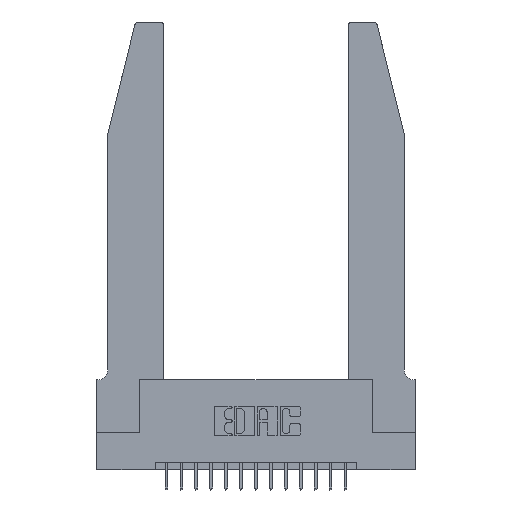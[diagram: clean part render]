
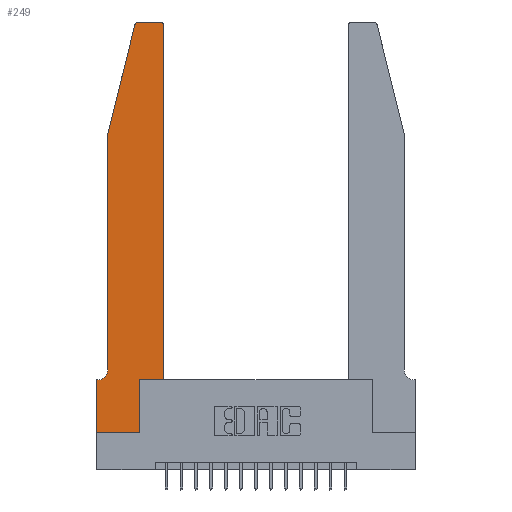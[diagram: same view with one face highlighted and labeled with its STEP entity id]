
A CAD part, top view. The second image highlights one B-rep face of the part: STEP entity #249.
In plain terms, the highlighted planar face has unit normal (0, 0, 1).
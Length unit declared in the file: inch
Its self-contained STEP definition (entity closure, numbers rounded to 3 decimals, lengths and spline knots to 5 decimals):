
#40 = CARTESIAN_POINT ( 'NONE',  ( 0., 0.35, 0.37 ) ) ;
#49 = ORIENTED_EDGE ( 'NONE', *, *, #11811, .T. ) ;
#57 = EDGE_CURVE ( 'NONE', #17818, #14148, #18195, .T. ) ;
#115 = EDGE_CURVE ( 'NONE', #15744, #13533, #5844, .T. ) ;
#156 = LINE ( 'NONE', #17797, #12013 ) ;
#249 = ADVANCED_FACE ( 'NONE', ( #4675 ), #346, .T. ) ;
#346 = PLANE ( 'NONE',  #12127 ) ;
#820 = VECTOR ( 'NONE', #7299, 39.37008 ) ;
#1170 = VERTEX_POINT ( 'NONE', #18199 ) ;
#1199 = ORIENTED_EDGE ( 'NONE', *, *, #8358, .T. ) ;
#1574 = CARTESIAN_POINT ( 'NONE',  ( 0.4205, 2.72, 0.37 ) ) ;
#1672 = VECTOR ( 'NONE', #6072, 39.37008 ) ;
#1860 = DIRECTION ( 'NONE',  ( 0., 0., 1. ) ) ;
#2452 = CARTESIAN_POINT ( 'NONE',  ( 0.4505, 0.35, 0.37 ) ) ;
#2607 = CIRCLE ( 'NONE', #3213, 0.07 ) ;
#2628 = CARTESIAN_POINT ( 'NONE',  ( 0.2865, 0.35, 0.37 ) ) ;
#2839 = ORIENTED_EDGE ( 'NONE', *, *, #11346, .T. ) ;
#3213 = AXIS2_PLACEMENT_3D ( 'NONE', #11190, #4967, #5063 ) ;
#3426 = DIRECTION ( 'NONE',  ( -1., 0., 0. ) ) ;
#3607 = VERTEX_POINT ( 'NONE', #10942 ) ;
#4304 = CARTESIAN_POINT ( 'NONE',  ( 0.0755, 0.35, 0.37 ) ) ;
#4504 = VECTOR ( 'NONE', #15338, 39.37008 ) ;
#4586 = DIRECTION ( 'NONE',  ( 0., -1., 0. ) ) ;
#4675 = FACE_OUTER_BOUND ( 'NONE', #10926, .T. ) ;
#4815 = CARTESIAN_POINT ( 'NONE',  ( 0.4505, 0.35, 0.37 ) ) ;
#4860 = VECTOR ( 'NONE', #8198, 39.37008 ) ;
#4967 = DIRECTION ( 'NONE',  ( 0., 0., -1. ) ) ;
#5063 = DIRECTION ( 'NONE',  ( -1., 0., 0. ) ) ;
#5079 = VECTOR ( 'NONE', #5709, 39.37008 ) ;
#5249 = LINE ( 'NONE', #2452, #4860 ) ;
#5508 = CARTESIAN_POINT ( 'NONE',  ( 0.284, 2.75, 0.37 ) ) ;
#5709 = DIRECTION ( 'NONE',  ( 0., 1., 0. ) ) ;
#5743 = CARTESIAN_POINT ( 'NONE',  ( 0.284, 2.72, 0.37 ) ) ;
#5776 = VERTEX_POINT ( 'NONE', #12564 ) ;
#5844 = LINE ( 'NONE', #4304, #6337 ) ;
#5943 = CARTESIAN_POINT ( 'NONE',  ( 0.2605, 2.75, 0.37 ) ) ;
#6072 = DIRECTION ( 'NONE',  ( 0., 1., 0. ) ) ;
#6212 = CARTESIAN_POINT ( 'NONE',  ( 0., 0.35, 0.37 ) ) ;
#6304 = DIRECTION ( 'NONE',  ( 0., 0., 1. ) ) ;
#6337 = VECTOR ( 'NONE', #7261, 39.37008 ) ;
#6484 = ORIENTED_EDGE ( 'NONE', *, *, #9832, .T. ) ;
#6557 = CIRCLE ( 'NONE', #16665, 0.03 ) ;
#6812 = VERTEX_POINT ( 'NONE', #14524 ) ;
#6919 = LINE ( 'NONE', #17461, #820 ) ;
#7261 = DIRECTION ( 'NONE',  ( -1., 0., 0. ) ) ;
#7299 = DIRECTION ( 'NONE',  ( 0., -1., 0. ) ) ;
#7694 = DIRECTION ( 'NONE',  ( 1., 0., 0. ) ) ;
#7710 = VERTEX_POINT ( 'NONE', #11313 ) ;
#8198 = DIRECTION ( 'NONE',  ( 1., 0., 0. ) ) ;
#8358 = EDGE_CURVE ( 'NONE', #11262, #8542, #13575, .T. ) ;
#8542 = VERTEX_POINT ( 'NONE', #5508 ) ;
#8931 = VECTOR ( 'NONE', #3426, 39.37008 ) ;
#8966 = ORIENTED_EDGE ( 'NONE', *, *, #14050, .T. ) ;
#9378 = CIRCLE ( 'NONE', #13646, 0.03 ) ;
#9672 = DIRECTION ( 'NONE',  ( 1., 0., 0. ) ) ;
#9832 = EDGE_CURVE ( 'NONE', #18386, #15744, #2607, .T. ) ;
#10201 = CARTESIAN_POINT ( 'NONE',  ( 0.25487, 2.72718, 0.37 ) ) ;
#10366 = EDGE_CURVE ( 'NONE', #6812, #5776, #15955, .T. ) ;
#10909 = CARTESIAN_POINT ( 'NONE',  ( 0.0755, 2., 0.37 ) ) ;
#10926 = EDGE_LOOP ( 'NONE', ( #1199, #13448, #11722, #13352, #6484, #11766, #13700, #8966, #16496, #2839, #18941, #49 ) ) ;
#10942 = CARTESIAN_POINT ( 'NONE',  ( 0.4505, 0.35, 0.37 ) ) ;
#11142 = VECTOR ( 'NONE', #9672, 39.37008 ) ;
#11190 = CARTESIAN_POINT ( 'NONE',  ( 0.0055, 0.42, 0.37 ) ) ;
#11262 = VERTEX_POINT ( 'NONE', #13270 ) ;
#11313 = CARTESIAN_POINT ( 'NONE',  ( 0., 0., 0.37 ) ) ;
#11346 = EDGE_CURVE ( 'NONE', #5776, #3607, #5249, .T. ) ;
#11722 = ORIENTED_EDGE ( 'NONE', *, *, #57, .T. ) ;
#11766 = ORIENTED_EDGE ( 'NONE', *, *, #115, .T. ) ;
#11811 = EDGE_CURVE ( 'NONE', #1170, #11262, #6557, .T. ) ;
#12013 = VECTOR ( 'NONE', #4586, 39.37008 ) ;
#12127 = AXIS2_PLACEMENT_3D ( 'NONE', #6212, #6304, #13570 ) ;
#12173 = EDGE_CURVE ( 'NONE', #3607, #1170, #17931, .T. ) ;
#12564 = CARTESIAN_POINT ( 'NONE',  ( 0.2865, 0.35, 0.37 ) ) ;
#12763 = CARTESIAN_POINT ( 'NONE',  ( 0.0055, 0.35, 0.37 ) ) ;
#12901 = DIRECTION ( 'NONE',  ( 0., 0., 1. ) ) ;
#13069 = EDGE_CURVE ( 'NONE', #13533, #7710, #156, .T. ) ;
#13270 = CARTESIAN_POINT ( 'NONE',  ( 0.4205, 2.75, 0.37 ) ) ;
#13352 = ORIENTED_EDGE ( 'NONE', *, *, #18071, .T. ) ;
#13448 = ORIENTED_EDGE ( 'NONE', *, *, #18549, .T. ) ;
#13533 = VERTEX_POINT ( 'NONE', #40 ) ;
#13570 = DIRECTION ( 'NONE',  ( 1., 0., 0. ) ) ;
#13575 = LINE ( 'NONE', #5943, #8931 ) ;
#13646 = AXIS2_PLACEMENT_3D ( 'NONE', #5743, #12901, #18857 ) ;
#13700 = ORIENTED_EDGE ( 'NONE', *, *, #13069, .T. ) ;
#14050 = EDGE_CURVE ( 'NONE', #7710, #6812, #18401, .T. ) ;
#14148 = VERTEX_POINT ( 'NONE', #15998 ) ;
#14524 = CARTESIAN_POINT ( 'NONE',  ( 0.2865, 0., 0.37 ) ) ;
#15338 = DIRECTION ( 'NONE',  ( -0.239, -0.971, 0. ) ) ;
#15345 = CARTESIAN_POINT ( 'NONE',  ( 0., 0., 0.37 ) ) ;
#15744 = VERTEX_POINT ( 'NONE', #12763 ) ;
#15955 = LINE ( 'NONE', #2628, #5079 ) ;
#15998 = CARTESIAN_POINT ( 'NONE',  ( 0.0755, 2., 0.37 ) ) ;
#16496 = ORIENTED_EDGE ( 'NONE', *, *, #10366, .T. ) ;
#16665 = AXIS2_PLACEMENT_3D ( 'NONE', #1574, #1860, #7694 ) ;
#17461 = CARTESIAN_POINT ( 'NONE',  ( 0.0755, 2., 0.37 ) ) ;
#17797 = CARTESIAN_POINT ( 'NONE',  ( 0., 0., 0.37 ) ) ;
#17818 = VERTEX_POINT ( 'NONE', #10201 ) ;
#17931 = LINE ( 'NONE', #4815, #1672 ) ;
#18071 = EDGE_CURVE ( 'NONE', #14148, #18386, #6919, .T. ) ;
#18195 = LINE ( 'NONE', #10909, #4504 ) ;
#18199 = CARTESIAN_POINT ( 'NONE',  ( 0.4505, 2.72, 0.37 ) ) ;
#18293 = CARTESIAN_POINT ( 'NONE',  ( 0.0755, 0.42, 0.37 ) ) ;
#18386 = VERTEX_POINT ( 'NONE', #18293 ) ;
#18401 = LINE ( 'NONE', #15345, #11142 ) ;
#18549 = EDGE_CURVE ( 'NONE', #8542, #17818, #9378, .T. ) ;
#18857 = DIRECTION ( 'NONE',  ( 1., 0., 0. ) ) ;
#18941 = ORIENTED_EDGE ( 'NONE', *, *, #12173, .T. ) ;
